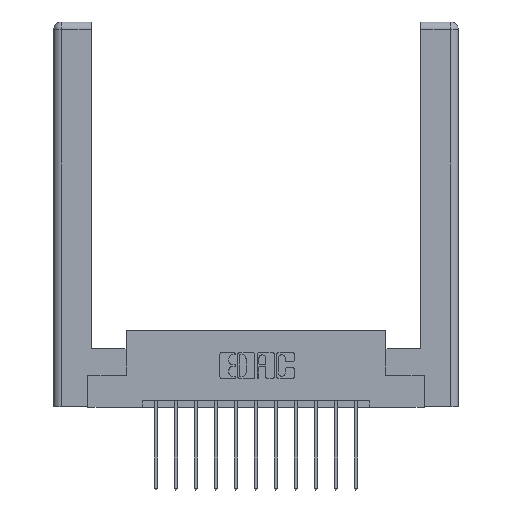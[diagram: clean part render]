
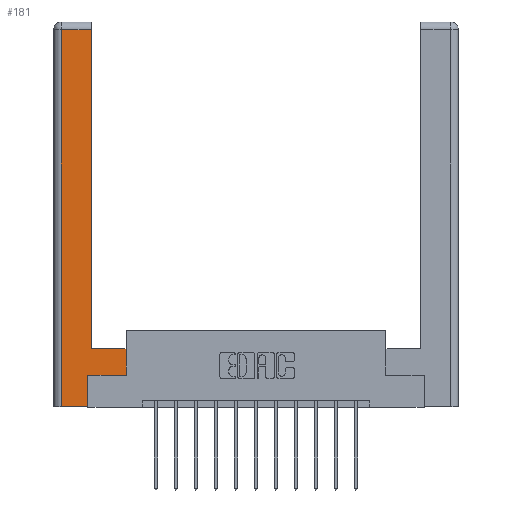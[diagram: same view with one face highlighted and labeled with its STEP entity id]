
A CAD part, top view. The second image highlights one B-rep face of the part: STEP entity #181.
In plain terms, the highlighted planar face has unit normal (0, 0, 1).
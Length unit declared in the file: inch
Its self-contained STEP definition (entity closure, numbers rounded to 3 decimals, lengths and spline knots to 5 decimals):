
#181 = ADVANCED_FACE ( 'NONE', ( #7611 ), #8750, .F. ) ;
#567 = LINE ( 'NONE', #9977, #2424 ) ;
#943 = ORIENTED_EDGE ( 'NONE', *, *, #12435, .T. ) ;
#1075 = DIRECTION ( 'NONE',  ( 0., 1., 0. ) ) ;
#1396 = ORIENTED_EDGE ( 'NONE', *, *, #5320, .T. ) ;
#1723 = DIRECTION ( 'NONE',  ( 0., 0., -1. ) ) ;
#1854 = LINE ( 'NONE', #7596, #2590 ) ;
#1869 = CARTESIAN_POINT ( 'NONE',  ( 0., 0., 0. ) ) ;
#1924 = DIRECTION ( 'NONE',  ( -1., 0., 0. ) ) ;
#2143 = EDGE_LOOP ( 'NONE', ( #4109, #11283, #3583, #3099, #943, #10426, #1396, #4743 ) ) ;
#2348 = VERTEX_POINT ( 'NONE', #11987 ) ;
#2424 = VECTOR ( 'NONE', #11133, 39.37008 ) ;
#2464 = CARTESIAN_POINT ( 'NONE',  ( 0.295, 2.94, 0. ) ) ;
#2470 = LINE ( 'NONE', #3065, #10360 ) ;
#2590 = VECTOR ( 'NONE', #9167, 39.37008 ) ;
#3065 = CARTESIAN_POINT ( 'NONE',  ( 0.0615, 2.94, 0. ) ) ;
#3099 = ORIENTED_EDGE ( 'NONE', *, *, #6046, .T. ) ;
#3514 = VERTEX_POINT ( 'NONE', #13261 ) ;
#3583 = ORIENTED_EDGE ( 'NONE', *, *, #5935, .T. ) ;
#3586 = CARTESIAN_POINT ( 'NONE',  ( 0.0615, 0., 0. ) ) ;
#3637 = VERTEX_POINT ( 'NONE', #15167 ) ;
#3638 = CARTESIAN_POINT ( 'NONE',  ( 0.565, 0.245, 0. ) ) ;
#3805 = DIRECTION ( 'NONE',  ( -1., 0., 0. ) ) ;
#4109 = ORIENTED_EDGE ( 'NONE', *, *, #4472, .T. ) ;
#4380 = DIRECTION ( 'NONE',  ( -1., 0., 0. ) ) ;
#4472 = EDGE_CURVE ( 'NONE', #3637, #10608, #6138, .T. ) ;
#4743 = ORIENTED_EDGE ( 'NONE', *, *, #7618, .T. ) ;
#4791 = VECTOR ( 'NONE', #12857, 39.37008 ) ;
#5320 = EDGE_CURVE ( 'NONE', #5654, #3514, #1854, .T. ) ;
#5532 = EDGE_CURVE ( 'NONE', #7514, #5654, #8449, .T. ) ;
#5654 = VERTEX_POINT ( 'NONE', #3638 ) ;
#5935 = EDGE_CURVE ( 'NONE', #2348, #15146, #12998, .T. ) ;
#6046 = EDGE_CURVE ( 'NONE', #15146, #10529, #10102, .T. ) ;
#6138 = LINE ( 'NONE', #8097, #14700 ) ;
#6437 = DIRECTION ( 'NONE',  ( 1., 0., 0. ) ) ;
#6508 = AXIS2_PLACEMENT_3D ( 'NONE', #1869, #1723, #1924 ) ;
#6824 = VECTOR ( 'NONE', #11759, 39.37008 ) ;
#6879 = CARTESIAN_POINT ( 'NONE',  ( 0.265, 0., 0. ) ) ;
#7030 = VECTOR ( 'NONE', #6437, 39.37008 ) ;
#7514 = VERTEX_POINT ( 'NONE', #14607 ) ;
#7596 = CARTESIAN_POINT ( 'NONE',  ( 0.565, 0.45, 0. ) ) ;
#7611 = FACE_OUTER_BOUND ( 'NONE', #2143, .T. ) ;
#7618 = EDGE_CURVE ( 'NONE', #3514, #3637, #13687, .T. ) ;
#8097 = CARTESIAN_POINT ( 'NONE',  ( 0.295, 3., 0. ) ) ;
#8449 = LINE ( 'NONE', #11142, #7030 ) ;
#8750 = PLANE ( 'NONE',  #6508 ) ;
#9167 = DIRECTION ( 'NONE',  ( 0., 1., 0. ) ) ;
#9306 = EDGE_CURVE ( 'NONE', #10608, #2348, #2470, .T. ) ;
#9977 = CARTESIAN_POINT ( 'NONE',  ( 0.265, 0.245, 0. ) ) ;
#10102 = LINE ( 'NONE', #6879, #4791 ) ;
#10360 = VECTOR ( 'NONE', #4380, 39.37008 ) ;
#10426 = ORIENTED_EDGE ( 'NONE', *, *, #5532, .T. ) ;
#10529 = VERTEX_POINT ( 'NONE', #13620 ) ;
#10608 = VERTEX_POINT ( 'NONE', #2464 ) ;
#11133 = DIRECTION ( 'NONE',  ( 0., 1., 0. ) ) ;
#11142 = CARTESIAN_POINT ( 'NONE',  ( 0.565, 0.245, 0. ) ) ;
#11283 = ORIENTED_EDGE ( 'NONE', *, *, #9306, .T. ) ;
#11759 = DIRECTION ( 'NONE',  ( 0., -1., 0. ) ) ;
#11987 = CARTESIAN_POINT ( 'NONE',  ( 0.0615, 2.94, 0. ) ) ;
#12435 = EDGE_CURVE ( 'NONE', #10529, #7514, #567, .T. ) ;
#12857 = DIRECTION ( 'NONE',  ( 1., 0., 0. ) ) ;
#12998 = LINE ( 'NONE', #3586, #6824 ) ;
#13261 = CARTESIAN_POINT ( 'NONE',  ( 0.565, 0.45, 0. ) ) ;
#13497 = VECTOR ( 'NONE', #3805, 39.37008 ) ;
#13620 = CARTESIAN_POINT ( 'NONE',  ( 0.265, 0., 0. ) ) ;
#13687 = LINE ( 'NONE', #14869, #13497 ) ;
#14481 = CARTESIAN_POINT ( 'NONE',  ( 0.0615, 0., 0. ) ) ;
#14607 = CARTESIAN_POINT ( 'NONE',  ( 0.265, 0.245, 0. ) ) ;
#14700 = VECTOR ( 'NONE', #1075, 39.37008 ) ;
#14869 = CARTESIAN_POINT ( 'NONE',  ( 0.295, 0.45, 0. ) ) ;
#15146 = VERTEX_POINT ( 'NONE', #14481 ) ;
#15167 = CARTESIAN_POINT ( 'NONE',  ( 0.295, 0.45, 0. ) ) ;
